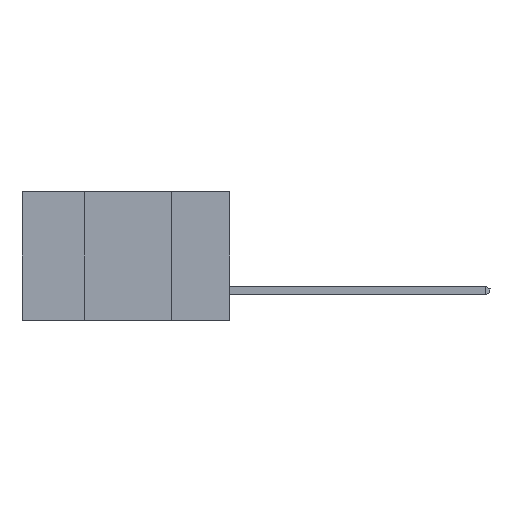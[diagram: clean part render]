
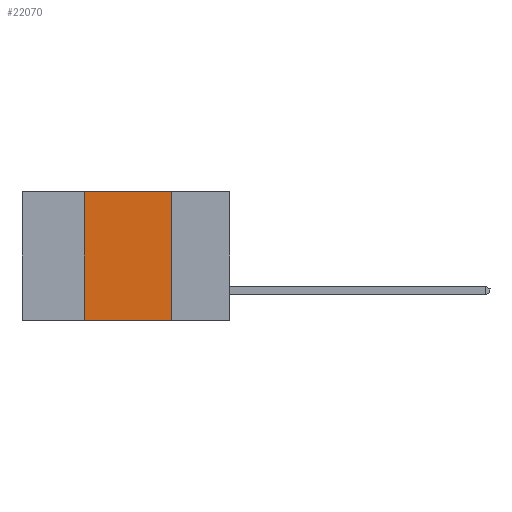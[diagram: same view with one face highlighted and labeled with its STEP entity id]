
A CAD part, left-side view. The second image highlights one B-rep face of the part: STEP entity #22070.
In plain terms, the highlighted planar face has unit normal (-1, 0, 0).
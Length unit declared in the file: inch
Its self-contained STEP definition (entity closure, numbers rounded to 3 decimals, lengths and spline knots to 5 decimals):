
#154 = VECTOR ( 'NONE', #4755, 39.37008 ) ;
#180 = ORIENTED_EDGE ( 'NONE', *, *, #9545, .F. ) ;
#499 = LINE ( 'NONE', #2325, #1792 ) ;
#810 = EDGE_CURVE ( 'NONE', #22055, #4209, #17048, .T. ) ;
#1225 = CARTESIAN_POINT ( 'NONE',  ( 0., 0.42, -0.37 ) ) ;
#1332 = ORIENTED_EDGE ( 'NONE', *, *, #15679, .F. ) ;
#1646 = ORIENTED_EDGE ( 'NONE', *, *, #18333, .T. ) ;
#1792 = VECTOR ( 'NONE', #14632, 39.37008 ) ;
#2325 = CARTESIAN_POINT ( 'NONE',  ( 0., 0.6, 0. ) ) ;
#2596 = DIRECTION ( 'NONE',  ( 0., 0., -1. ) ) ;
#3105 = FACE_OUTER_BOUND ( 'NONE', #16050, .T. ) ;
#3215 = CARTESIAN_POINT ( 'NONE',  ( 0., 0.42, -0.37 ) ) ;
#4209 = VERTEX_POINT ( 'NONE', #13619 ) ;
#4342 = VECTOR ( 'NONE', #21385, 39.37008 ) ;
#4755 = DIRECTION ( 'NONE',  ( 0., 0., 1. ) ) ;
#5329 = ORIENTED_EDGE ( 'NONE', *, *, #810, .F. ) ;
#5791 = LINE ( 'NONE', #20096, #18749 ) ;
#5848 = VERTEX_POINT ( 'NONE', #7920 ) ;
#7920 = CARTESIAN_POINT ( 'NONE',  ( 0., 0.17, 0. ) ) ;
#8441 = DIRECTION ( 'NONE',  ( 1., 0., 0. ) ) ;
#9545 = EDGE_CURVE ( 'NONE', #4209, #5848, #499, .T. ) ;
#9832 = DIRECTION ( 'NONE',  ( 0., 0., -1. ) ) ;
#10156 = CARTESIAN_POINT ( 'NONE',  ( 0., 0.6, 0. ) ) ;
#13619 = CARTESIAN_POINT ( 'NONE',  ( 0., 0.42, 0. ) ) ;
#14632 = DIRECTION ( 'NONE',  ( 0., -1., 0. ) ) ;
#14779 = CARTESIAN_POINT ( 'NONE',  ( 0., 0.17, -0.37 ) ) ;
#15679 = EDGE_CURVE ( 'NONE', #5848, #17389, #5791, .T. ) ;
#16050 = EDGE_LOOP ( 'NONE', ( #1332, #180, #5329, #1646 ) ) ;
#16182 = CARTESIAN_POINT ( 'NONE',  ( 0., 0.6, -0.37 ) ) ;
#16483 = AXIS2_PLACEMENT_3D ( 'NONE', #10156, #8441, #9832 ) ;
#17048 = LINE ( 'NONE', #1225, #154 ) ;
#17389 = VERTEX_POINT ( 'NONE', #14779 ) ;
#17886 = LINE ( 'NONE', #16182, #4342 ) ;
#18333 = EDGE_CURVE ( 'NONE', #22055, #17389, #17886, .T. ) ;
#18749 = VECTOR ( 'NONE', #2596, 39.37008 ) ;
#20096 = CARTESIAN_POINT ( 'NONE',  ( 0., 0.17, -0.37 ) ) ;
#20484 = PLANE ( 'NONE',  #16483 ) ;
#21385 = DIRECTION ( 'NONE',  ( 0., -1., 0. ) ) ;
#22055 = VERTEX_POINT ( 'NONE', #3215 ) ;
#22070 = ADVANCED_FACE ( 'NONE', ( #3105 ), #20484, .F. ) ;
